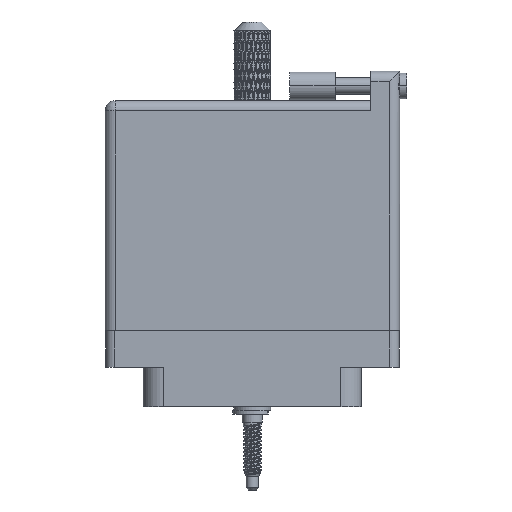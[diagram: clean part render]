
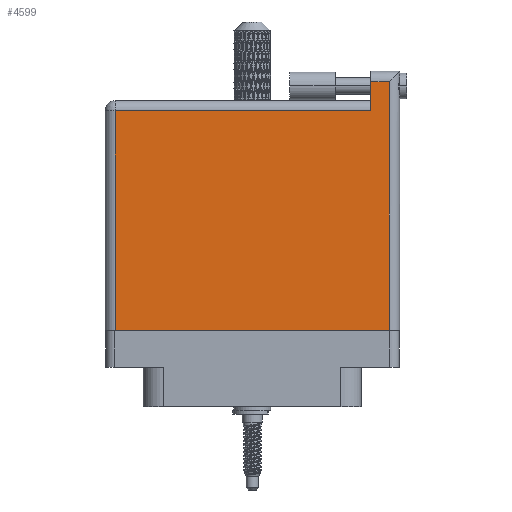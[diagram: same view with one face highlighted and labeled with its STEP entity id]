
A CAD part, front view. The second image highlights one B-rep face of the part: STEP entity #4599.
In plain terms, the highlighted face is planar.
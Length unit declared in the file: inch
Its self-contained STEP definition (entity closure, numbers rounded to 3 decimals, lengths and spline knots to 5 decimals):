
#2534 = EDGE_CURVE ( 'NONE', #62584, #24069, #11546, .T. ) ;
#4599 = ADVANCED_FACE ( 'NONE', ( #15346 ), #47807, .F. ) ;
#6218 = VERTEX_POINT ( 'NONE', #36721 ) ;
#10430 = CARTESIAN_POINT ( 'NONE',  ( -0.934, -0.1, 0.4495 ) ) ;
#10813 = DIRECTION ( 'NONE',  ( 0., 1., 0. ) ) ;
#11454 = EDGE_CURVE ( 'NONE', #24069, #6218, #77492, .T. ) ;
#11546 = LINE ( 'NONE', #10430, #19248 ) ;
#13128 = CARTESIAN_POINT ( 'NONE',  ( -1.004, 1.396, 0.4495 ) ) ;
#13641 = ORIENTED_EDGE ( 'NONE', *, *, #25069, .T. ) ;
#14306 = AXIS2_PLACEMENT_3D ( 'NONE', #23491, #80655, #57733 ) ;
#15174 = EDGE_CURVE ( 'NONE', #43249, #62584, #68149, .T. ) ;
#15346 = FACE_OUTER_BOUND ( 'NONE', #36279, .T. ) ;
#19179 = DIRECTION ( 'NONE',  ( 1., 0., 0. ) ) ;
#19248 = VECTOR ( 'NONE', #75720, 39.37008 ) ;
#23491 = CARTESIAN_POINT ( 'NONE',  ( -1.004, 1.466, 0.4495 ) ) ;
#24069 = VERTEX_POINT ( 'NONE', #37852 ) ;
#25069 = EDGE_CURVE ( 'NONE', #103317, #43249, #82505, .T. ) ;
#25622 = ORIENTED_EDGE ( 'NONE', *, *, #2534, .T. ) ;
#32285 = CARTESIAN_POINT ( 'NONE',  ( 0.807, 1.596, 0.4495 ) ) ;
#35006 = VECTOR ( 'NONE', #104031, 39.37008 ) ;
#36279 = EDGE_LOOP ( 'NONE', ( #43460, #61549, #50405, #13641, #93127, #25622 ) ) ;
#36721 = CARTESIAN_POINT ( 'NONE',  ( 0.934, -0.1, 0.4495 ) ) ;
#37852 = CARTESIAN_POINT ( 'NONE',  ( -0.934, -0.1, 0.4495 ) ) ;
#43249 = VERTEX_POINT ( 'NONE', #69131 ) ;
#43460 = ORIENTED_EDGE ( 'NONE', *, *, #11454, .T. ) ;
#43908 = LINE ( 'NONE', #78364, #35006 ) ;
#45507 = VECTOR ( 'NONE', #19179, 39.37008 ) ;
#46373 = DIRECTION ( 'NONE',  ( 0., -1., 0. ) ) ;
#47807 = PLANE ( 'NONE',  #14306 ) ;
#50405 = ORIENTED_EDGE ( 'NONE', *, *, #98148, .T. ) ;
#54222 = DIRECTION ( 'NONE',  ( -1., 0., 0. ) ) ;
#54952 = CARTESIAN_POINT ( 'NONE',  ( 0.807, 1.666, 0.4495 ) ) ;
#57733 = DIRECTION ( 'NONE',  ( -1., 0., 0. ) ) ;
#59705 = CARTESIAN_POINT ( 'NONE',  ( 0.934, 1.666, 0.4495 ) ) ;
#61549 = ORIENTED_EDGE ( 'NONE', *, *, #65819, .T. ) ;
#61880 = VECTOR ( 'NONE', #10813, 39.37008 ) ;
#62584 = VERTEX_POINT ( 'NONE', #70207 ) ;
#65819 = EDGE_CURVE ( 'NONE', #6218, #97928, #91321, .T. ) ;
#68149 = LINE ( 'NONE', #13128, #105251 ) ;
#69131 = CARTESIAN_POINT ( 'NONE',  ( 0.807, 1.396, 0.4495 ) ) ;
#70207 = CARTESIAN_POINT ( 'NONE',  ( -0.934, 1.396, 0.4495 ) ) ;
#73850 = CARTESIAN_POINT ( 'NONE',  ( 0.934, 1.596, 0.4495 ) ) ;
#75720 = DIRECTION ( 'NONE',  ( 0., -1., 0. ) ) ;
#77492 = LINE ( 'NONE', #100578, #45507 ) ;
#78364 = CARTESIAN_POINT ( 'NONE',  ( -1.004, 1.596, 0.4495 ) ) ;
#80655 = DIRECTION ( 'NONE',  ( 0., 0., -1. ) ) ;
#82505 = LINE ( 'NONE', #54952, #96592 ) ;
#91321 = LINE ( 'NONE', #59705, #61880 ) ;
#93127 = ORIENTED_EDGE ( 'NONE', *, *, #15174, .T. ) ;
#96592 = VECTOR ( 'NONE', #46373, 39.37008 ) ;
#97928 = VERTEX_POINT ( 'NONE', #73850 ) ;
#98148 = EDGE_CURVE ( 'NONE', #97928, #103317, #43908, .T. ) ;
#100578 = CARTESIAN_POINT ( 'NONE',  ( -1.004, -0.1, 0.4495 ) ) ;
#103317 = VERTEX_POINT ( 'NONE', #32285 ) ;
#104031 = DIRECTION ( 'NONE',  ( -1., 0., 0. ) ) ;
#105251 = VECTOR ( 'NONE', #54222, 39.37008 ) ;
